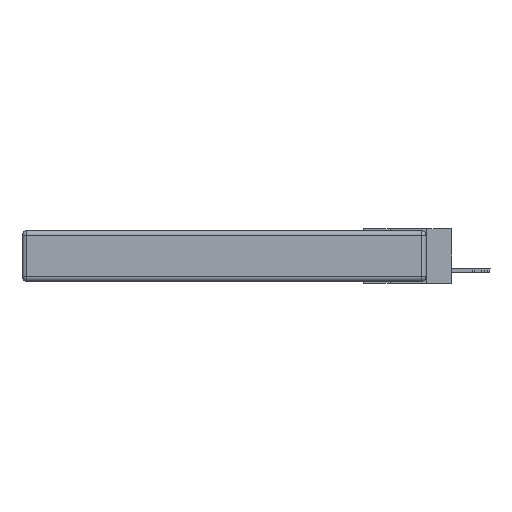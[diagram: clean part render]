
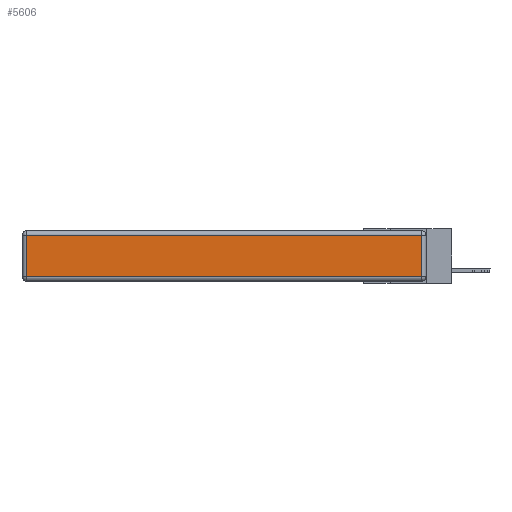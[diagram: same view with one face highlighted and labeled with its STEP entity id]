
A CAD part, left-side view. The second image highlights one B-rep face of the part: STEP entity #5606.
In plain terms, the highlighted planar face has unit normal (-1, 0, 0).
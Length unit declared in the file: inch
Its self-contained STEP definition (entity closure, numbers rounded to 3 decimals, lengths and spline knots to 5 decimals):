
#157 = EDGE_LOOP ( 'NONE', ( #16844, #28026, #6116, #30269 ) ) ;
#3061 = VERTEX_POINT ( 'NONE', #26610 ) ;
#3381 = EDGE_CURVE ( 'NONE', #3061, #10027, #32018, .T. ) ;
#5530 = CARTESIAN_POINT ( 'NONE',  ( 0., 0., -0.313 ) ) ;
#5606 = ADVANCED_FACE ( 'NONE', ( #17728 ), #19909, .T. ) ;
#6116 = ORIENTED_EDGE ( 'NONE', *, *, #10756, .T. ) ;
#6833 = VERTEX_POINT ( 'NONE', #10546 ) ;
#7985 = VECTOR ( 'NONE', #12815, 39.37008 ) ;
#8073 = CARTESIAN_POINT ( 'NONE',  ( 0., 2.72, -0.313 ) ) ;
#9678 = DIRECTION ( 'NONE',  ( -1., 0., 0. ) ) ;
#10027 = VERTEX_POINT ( 'NONE', #8073 ) ;
#10546 = CARTESIAN_POINT ( 'NONE',  ( 0., 0.03, -0.03 ) ) ;
#10756 = EDGE_CURVE ( 'NONE', #6833, #3061, #20737, .T. ) ;
#11609 = CARTESIAN_POINT ( 'NONE',  ( 0., 0.03, -0.313 ) ) ;
#12815 = DIRECTION ( 'NONE',  ( 0., 1., 0. ) ) ;
#15968 = LINE ( 'NONE', #5530, #20910 ) ;
#16844 = ORIENTED_EDGE ( 'NONE', *, *, #16945, .T. ) ;
#16945 = EDGE_CURVE ( 'NONE', #10027, #29440, #15968, .T. ) ;
#17377 = DIRECTION ( 'NONE',  ( 0., 0., 1. ) ) ;
#17728 = FACE_OUTER_BOUND ( 'NONE', #157, .T. ) ;
#18155 = LINE ( 'NONE', #24569, #20646 ) ;
#19909 = PLANE ( 'NONE',  #26756 ) ;
#20646 = VECTOR ( 'NONE', #27460, 39.37008 ) ;
#20737 = LINE ( 'NONE', #28613, #7985 ) ;
#20910 = VECTOR ( 'NONE', #26485, 39.37008 ) ;
#20999 = EDGE_CURVE ( 'NONE', #29440, #6833, #18155, .T. ) ;
#24569 = CARTESIAN_POINT ( 'NONE',  ( 0., 0.03, -0.343 ) ) ;
#25778 = DIRECTION ( 'NONE',  ( 0., 0., -1. ) ) ;
#25995 = CARTESIAN_POINT ( 'NONE',  ( 0., 2.72, -0.343 ) ) ;
#26485 = DIRECTION ( 'NONE',  ( 0., -1., 0. ) ) ;
#26610 = CARTESIAN_POINT ( 'NONE',  ( 0., 2.72, -0.03 ) ) ;
#26756 = AXIS2_PLACEMENT_3D ( 'NONE', #32904, #9678, #17377 ) ;
#27460 = DIRECTION ( 'NONE',  ( 0., 0., 1. ) ) ;
#28026 = ORIENTED_EDGE ( 'NONE', *, *, #20999, .T. ) ;
#28613 = CARTESIAN_POINT ( 'NONE',  ( 0., 2.75, -0.03 ) ) ;
#29440 = VERTEX_POINT ( 'NONE', #11609 ) ;
#30269 = ORIENTED_EDGE ( 'NONE', *, *, #3381, .T. ) ;
#30786 = VECTOR ( 'NONE', #25778, 39.37008 ) ;
#32018 = LINE ( 'NONE', #25995, #30786 ) ;
#32904 = CARTESIAN_POINT ( 'NONE',  ( 0., 0., -0.343 ) ) ;
